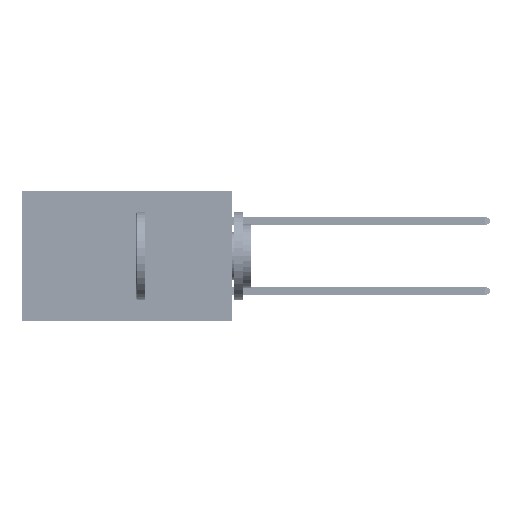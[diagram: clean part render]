
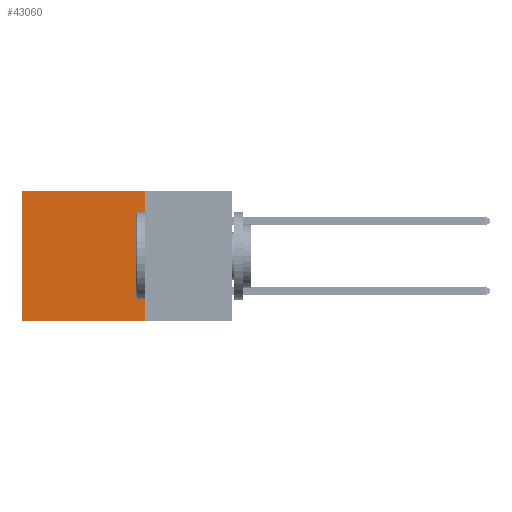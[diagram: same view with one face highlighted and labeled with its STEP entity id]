
A CAD part, left-side view. The second image highlights one B-rep face of the part: STEP entity #43060.
In plain terms, the highlighted planar face has unit normal (-1, 0, 0).
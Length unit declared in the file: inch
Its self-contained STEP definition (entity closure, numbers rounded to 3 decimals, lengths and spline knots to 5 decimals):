
#2725 = CARTESIAN_POINT ( 'NONE',  ( 0.2875, 0.25, -0.37 ) ) ;
#3009 = VECTOR ( 'NONE', #6015, 39.37008 ) ;
#4076 = DIRECTION ( 'NONE',  ( 0., 0., -1. ) ) ;
#4190 = CARTESIAN_POINT ( 'NONE',  ( 0.2875, 0.25, -0.37 ) ) ;
#4826 = EDGE_CURVE ( 'NONE', #32457, #19247, #40035, .T. ) ;
#5765 = VERTEX_POINT ( 'NONE', #2725 ) ;
#6015 = DIRECTION ( 'NONE',  ( 0., 0., -1. ) ) ;
#6657 = EDGE_CURVE ( 'NONE', #5765, #19247, #40999, .T. ) ;
#9348 = VECTOR ( 'NONE', #4076, 39.37008 ) ;
#10934 = CARTESIAN_POINT ( 'NONE',  ( 0.2875, 0.25, 0. ) ) ;
#12699 = VERTEX_POINT ( 'NONE', #20280 ) ;
#18079 = VECTOR ( 'NONE', #20335, 39.37008 ) ;
#19247 = VERTEX_POINT ( 'NONE', #19484 ) ;
#19484 = CARTESIAN_POINT ( 'NONE',  ( 0.2875, 0.6, -0.37 ) ) ;
#20280 = CARTESIAN_POINT ( 'NONE',  ( 0.2875, 0.25, 0. ) ) ;
#20335 = DIRECTION ( 'NONE',  ( 0., 1., 0. ) ) ;
#23564 = AXIS2_PLACEMENT_3D ( 'NONE', #37052, #25250, #41253 ) ;
#25250 = DIRECTION ( 'NONE',  ( 1., 0., 0. ) ) ;
#25520 = ORIENTED_EDGE ( 'NONE', *, *, #26759, .T. ) ;
#26596 = LINE ( 'NONE', #10934, #30184 ) ;
#26759 = EDGE_CURVE ( 'NONE', #12699, #32457, #26596, .T. ) ;
#27112 = CARTESIAN_POINT ( 'NONE',  ( 0.2875, 0.6, 0. ) ) ;
#28498 = EDGE_CURVE ( 'NONE', #12699, #5765, #47016, .T. ) ;
#29269 = PLANE ( 'NONE',  #23564 ) ;
#30184 = VECTOR ( 'NONE', #37861, 39.37008 ) ;
#32457 = VERTEX_POINT ( 'NONE', #32621 ) ;
#32621 = CARTESIAN_POINT ( 'NONE',  ( 0.2875, 0.6, 0. ) ) ;
#33409 = CARTESIAN_POINT ( 'NONE',  ( 0.2875, 0.25, 0. ) ) ;
#33857 = EDGE_LOOP ( 'NONE', ( #44123, #44440, #49583, #25520 ) ) ;
#37052 = CARTESIAN_POINT ( 'NONE',  ( 0.2875, 0.25, 0. ) ) ;
#37861 = DIRECTION ( 'NONE',  ( 0., 1., 0. ) ) ;
#40035 = LINE ( 'NONE', #27112, #9348 ) ;
#40999 = LINE ( 'NONE', #4190, #18079 ) ;
#41253 = DIRECTION ( 'NONE',  ( 0., 0., -1. ) ) ;
#43060 = ADVANCED_FACE ( 'NONE', ( #44558 ), #29269, .F. ) ;
#44123 = ORIENTED_EDGE ( 'NONE', *, *, #4826, .T. ) ;
#44440 = ORIENTED_EDGE ( 'NONE', *, *, #6657, .F. ) ;
#44558 = FACE_OUTER_BOUND ( 'NONE', #33857, .T. ) ;
#47016 = LINE ( 'NONE', #33409, #3009 ) ;
#49583 = ORIENTED_EDGE ( 'NONE', *, *, #28498, .F. ) ;
